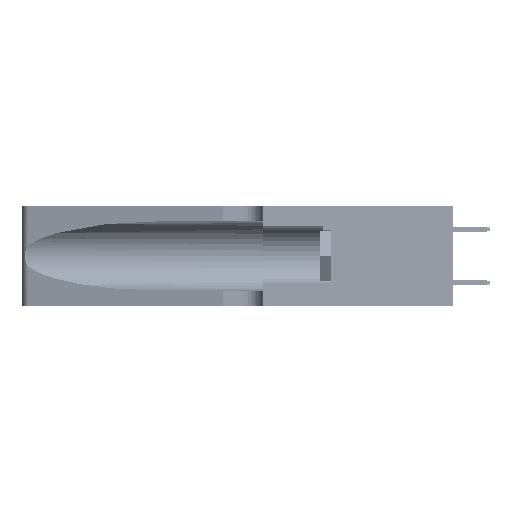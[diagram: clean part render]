
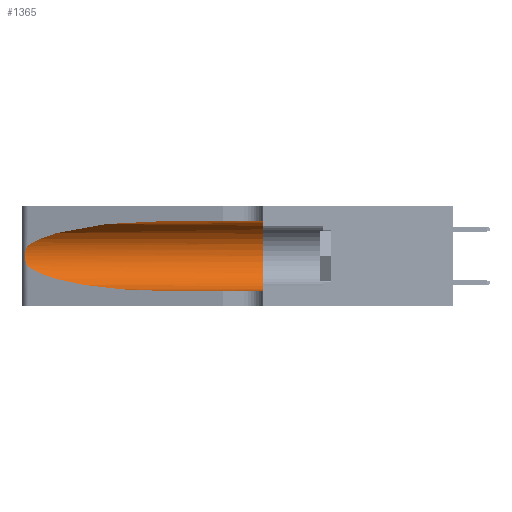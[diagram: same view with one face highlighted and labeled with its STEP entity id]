
A CAD part, left-side view. The second image highlights one B-rep face of the part: STEP entity #1365.
In plain terms, the highlighted cylindrical face has radius 3.308 mm (diameter 6.617 mm), a partial arc.
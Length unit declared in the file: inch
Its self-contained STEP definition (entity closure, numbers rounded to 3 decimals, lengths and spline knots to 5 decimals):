
#73 = VERTEX_POINT ( 'NONE', #43041 ) ;
#369 = CARTESIAN_POINT ( 'NONE',  ( 0.2373, 1.15595, 0.08982 ) ) ;
#1126 = AXIS2_PLACEMENT_3D ( 'NONE', #31860, #18423, #51899 ) ;
#1365 = ADVANCED_FACE ( 'NONE', ( #14241 ), #30965, .F. ) ;
#2017 = VERTEX_POINT ( 'NONE', #2655 ) ;
#2655 = CARTESIAN_POINT ( 'NONE',  ( 0.1305, 0.72297, 0.31525 ) ) ;
#2796 = EDGE_CURVE ( 'NONE', #15656, #6974, #13572, .T. ) ;
#2862 = CIRCLE ( 'NONE', #1126, 0.13025 ) ;
#3076 = CARTESIAN_POINT ( 'NONE',  ( 0.25555, 1.22993, 0.14849 ) ) ;
#4681 = CARTESIAN_POINT ( 'NONE',  ( 0.1305, 1.61858, 0.31525 ) ) ;
#5305 = ORIENTED_EDGE ( 'NONE', *, *, #48314, .T. ) ;
#6974 = VERTEX_POINT ( 'NONE', #24672 ) ;
#7015 = VECTOR ( 'NONE', #34054, 39.37008 ) ;
#9429 = ORIENTED_EDGE ( 'NONE', *, *, #2796, .T. ) ;
#10645 = ORIENTED_EDGE ( 'NONE', *, *, #37467, .F. ) ;
#13273 = EDGE_LOOP ( 'NONE', ( #5305, #9429, #46438, #15978, #31845, #10645 ) ) ;
#13572 = B_SPLINE_CURVE_WITH_KNOTS ( 'NONE', 3,
 ( #15128, #48608, #40100, #44495, #32419, #23363, #23618, #23889, #28275, #27995, #23076, #40644, #3076, #35719 ),
 .UNSPECIFIED., .F., .F.,
 ( 4, 2, 2, 2, 2, 2, 4 ),
 ( 0., 0.00027, 0.00053, 0.00107, 0.0016, 0.00187, 0.00214 ),
 .UNSPECIFIED. ) ;
#14229 = EDGE_CURVE ( 'NONE', #73, #22511, #15620, .T. ) ;
#14241 = FACE_OUTER_BOUND ( 'NONE', #13273, .T. ) ;
#15128 = CARTESIAN_POINT ( 'NONE',  ( 0.25487, 1.22718, 0.22369 ) ) ;
#15427 = CARTESIAN_POINT ( 'NONE',  ( 0.1305, 0.72297, 0.31525 ) ) ;
#15620 = LINE ( 'NONE', #19717, #46505 ) ;
#15656 = VERTEX_POINT ( 'NONE', #19896 ) ;
#15978 = ORIENTED_EDGE ( 'NONE', *, *, #14229, .T. ) ;
#16214 = CARTESIAN_POINT ( 'NONE',  ( 0.1305, 0.35, 0.05475 ) ) ;
#18423 = DIRECTION ( 'NONE',  ( 0., 1., 0. ) ) ;
#18479 = VERTEX_POINT ( 'NONE', #32347 ) ;
#19717 = CARTESIAN_POINT ( 'NONE',  ( 0.1305, 1.61858, 0.05475 ) ) ;
#19896 = CARTESIAN_POINT ( 'NONE',  ( 0.25487, 1.22718, 0.22369 ) ) ;
#22511 = VERTEX_POINT ( 'NONE', #16214 ) ;
#23076 = CARTESIAN_POINT ( 'NONE',  ( 0.25789, 1.23486, 0.15765 ) ) ;
#23363 = CARTESIAN_POINT ( 'NONE',  ( 0.26018, 1.23835, 0.19895 ) ) ;
#23618 = CARTESIAN_POINT ( 'NONE',  ( 0.26075, 1.23896, 0.19203 ) ) ;
#23639 = CARTESIAN_POINT ( 'NONE',  ( 0.25487, 1.22718, 0.22369 ) ) ;
#23889 = CARTESIAN_POINT ( 'NONE',  ( 0.26075, 1.23896, 0.178 ) ) ;
#24672 = CARTESIAN_POINT ( 'NONE',  ( 0.25487, 1.22718, 0.14631 ) ) ;
#27107 = CARTESIAN_POINT ( 'NONE',  ( 0.1305, 1.61858, 0.185 ) ) ;
#27151 =( BOUNDED_CURVE ( )  B_SPLINE_CURVE ( 3, ( #45373, #369, #33299, #50025 ),
 .UNSPECIFIED., .F., .F. ) 
 B_SPLINE_CURVE_WITH_KNOTS ( ( 4, 4 ),
 ( 3.44316, 4.71239 ),
 .UNSPECIFIED. ) 
 CURVE ( )  GEOMETRIC_REPRESENTATION_ITEM ( )  RATIONAL_B_SPLINE_CURVE ( ( 1., 0.87, 0.87, 1. ) ) 
 REPRESENTATION_ITEM ( '' )  );
#27995 = CARTESIAN_POINT ( 'NONE',  ( 0.25856, 1.23593, 0.16098 ) ) ;
#28275 = CARTESIAN_POINT ( 'NONE',  ( 0.26017, 1.23833, 0.17102 ) ) ;
#29079 = LINE ( 'NONE', #4681, #7015 ) ;
#30965 = CYLINDRICAL_SURFACE ( 'NONE', #41437, 0.13025 ) ;
#31845 = ORIENTED_EDGE ( 'NONE', *, *, #50736, .F. ) ;
#31860 = CARTESIAN_POINT ( 'NONE',  ( 0.1305, 0.35, 0.185 ) ) ;
#32347 = CARTESIAN_POINT ( 'NONE',  ( 0.1305, 0.35, 0.31525 ) ) ;
#32360 = DIRECTION ( 'NONE',  ( 0., -1., 0. ) ) ;
#32419 = CARTESIAN_POINT ( 'NONE',  ( 0.25854, 1.2359, 0.20912 ) ) ;
#33299 = CARTESIAN_POINT ( 'NONE',  ( 0.18966, 0.96281, 0.05475 ) ) ;
#34054 = DIRECTION ( 'NONE',  ( 0., -1., 0. ) ) ;
#35177 = CARTESIAN_POINT ( 'NONE',  ( 0.18966, 0.96281, 0.31525 ) ) ;
#35719 = CARTESIAN_POINT ( 'NONE',  ( 0.25487, 1.22718, 0.14631 ) ) ;
#37467 = EDGE_CURVE ( 'NONE', #2017, #18479, #29079, .T. ) ;
#40100 = CARTESIAN_POINT ( 'NONE',  ( 0.25639, 1.23184, 0.21858 ) ) ;
#40644 = CARTESIAN_POINT ( 'NONE',  ( 0.25639, 1.23186, 0.15144 ) ) ;
#41437 = AXIS2_PLACEMENT_3D ( 'NONE', #27107, #43870, #44149 ) ;
#43041 = CARTESIAN_POINT ( 'NONE',  ( 0.1305, 0.72297, 0.05475 ) ) ;
#43870 = DIRECTION ( 'NONE',  ( 0., -1., 0. ) ) ;
#44149 = DIRECTION ( 'NONE',  ( 0., 0., -1. ) ) ;
#44248 = CARTESIAN_POINT ( 'NONE',  ( 0.2373, 1.15595, 0.28018 ) ) ;
#44495 = CARTESIAN_POINT ( 'NONE',  ( 0.25787, 1.23484, 0.2124 ) ) ;
#45373 = CARTESIAN_POINT ( 'NONE',  ( 0.25487, 1.22718, 0.14631 ) ) ;
#45758 =( BOUNDED_CURVE ( )  B_SPLINE_CURVE ( 3, ( #15427, #35177, #44248, #23639 ),
 .UNSPECIFIED., .F., .T. ) 
 B_SPLINE_CURVE_WITH_KNOTS ( ( 4, 4 ),
 ( 1.5708, 2.84003 ),
 .UNSPECIFIED. ) 
 CURVE ( )  GEOMETRIC_REPRESENTATION_ITEM ( )  RATIONAL_B_SPLINE_CURVE ( ( 1., 0.87, 0.87, 1. ) ) 
 REPRESENTATION_ITEM ( '' )  );
#46438 = ORIENTED_EDGE ( 'NONE', *, *, #52436, .T. ) ;
#46505 = VECTOR ( 'NONE', #32360, 39.37008 ) ;
#48314 = EDGE_CURVE ( 'NONE', #2017, #15656, #45758, .T. ) ;
#48608 = CARTESIAN_POINT ( 'NONE',  ( 0.25555, 1.22994, 0.2215 ) ) ;
#50025 = CARTESIAN_POINT ( 'NONE',  ( 0.1305, 0.72297, 0.05475 ) ) ;
#50736 = EDGE_CURVE ( 'NONE', #18479, #22511, #2862, .T. ) ;
#51899 = DIRECTION ( 'NONE',  ( 0., 0., 1. ) ) ;
#52436 = EDGE_CURVE ( 'NONE', #6974, #73, #27151, .T. ) ;
